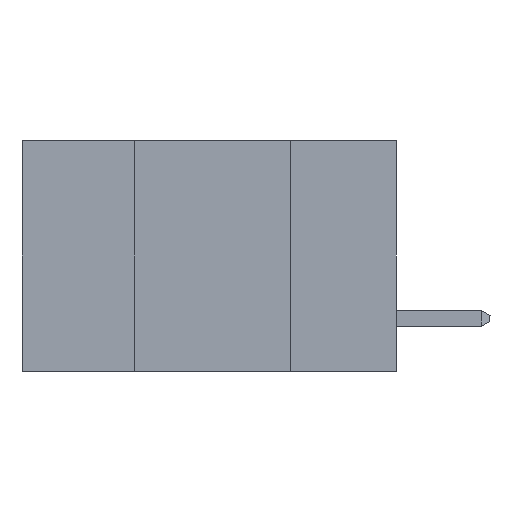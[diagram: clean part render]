
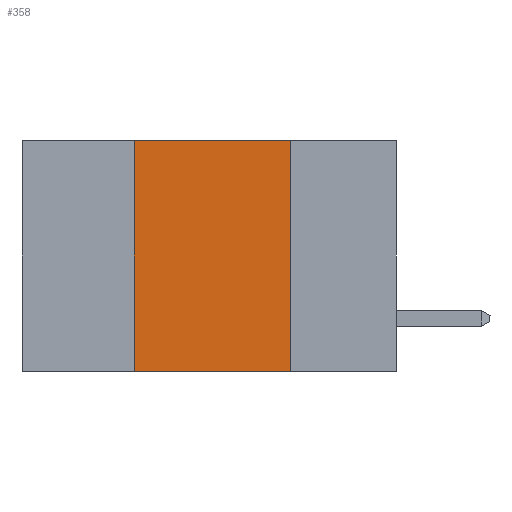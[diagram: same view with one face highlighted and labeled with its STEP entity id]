
A CAD part, left-side view. The second image highlights one B-rep face of the part: STEP entity #358.
In plain terms, the highlighted planar face has unit normal (-1, 0, 0).
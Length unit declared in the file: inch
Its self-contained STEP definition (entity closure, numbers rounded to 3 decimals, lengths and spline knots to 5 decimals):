
#358 = ADVANCED_FACE ( 'NONE', ( #4982 ), #2675, .F. ) ;
#968 = ORIENTED_EDGE ( 'NONE', *, *, #7099, .T. ) ;
#1927 = CARTESIAN_POINT ( 'NONE',  ( 0., 0.17, -0.37 ) ) ;
#2008 = CARTESIAN_POINT ( 'NONE',  ( 0., 0.6, -0.37 ) ) ;
#2015 = EDGE_CURVE ( 'NONE', #12877, #10382, #12241, .T. ) ;
#2230 = DIRECTION ( 'NONE',  ( 0., 0., 1. ) ) ;
#2251 = DIRECTION ( 'NONE',  ( 1., 0., 0. ) ) ;
#2473 = ORIENTED_EDGE ( 'NONE', *, *, #2015, .F. ) ;
#2675 = PLANE ( 'NONE',  #3673 ) ;
#2686 = CARTESIAN_POINT ( 'NONE',  ( 0., 0.17, 0. ) ) ;
#2893 = VERTEX_POINT ( 'NONE', #8122 ) ;
#3106 = DIRECTION ( 'NONE',  ( 0., -1., 0. ) ) ;
#3188 = CARTESIAN_POINT ( 'NONE',  ( 0., 0.42, -0.37 ) ) ;
#3673 = AXIS2_PLACEMENT_3D ( 'NONE', #11210, #2251, #12007 ) ;
#4173 = LINE ( 'NONE', #2008, #9363 ) ;
#4434 = LINE ( 'NONE', #12278, #9606 ) ;
#4982 = FACE_OUTER_BOUND ( 'NONE', #12709, .T. ) ;
#6560 = EDGE_CURVE ( 'NONE', #10850, #2893, #7350, .T. ) ;
#7099 = EDGE_CURVE ( 'NONE', #12877, #2893, #4173, .T. ) ;
#7350 = LINE ( 'NONE', #1927, #12438 ) ;
#7653 = ORIENTED_EDGE ( 'NONE', *, *, #9273, .F. ) ;
#8122 = CARTESIAN_POINT ( 'NONE',  ( 0., 0.17, -0.37 ) ) ;
#8143 = CARTESIAN_POINT ( 'NONE',  ( 0., 0.42, 0. ) ) ;
#8172 = DIRECTION ( 'NONE',  ( 0., 0., -1. ) ) ;
#9273 = EDGE_CURVE ( 'NONE', #10382, #10850, #4434, .T. ) ;
#9363 = VECTOR ( 'NONE', #3106, 39.37008 ) ;
#9596 = VECTOR ( 'NONE', #2230, 39.37008 ) ;
#9606 = VECTOR ( 'NONE', #11286, 39.37008 ) ;
#10382 = VERTEX_POINT ( 'NONE', #8143 ) ;
#10850 = VERTEX_POINT ( 'NONE', #2686 ) ;
#11210 = CARTESIAN_POINT ( 'NONE',  ( 0., 0.6, 0. ) ) ;
#11286 = DIRECTION ( 'NONE',  ( 0., -1., 0. ) ) ;
#12007 = DIRECTION ( 'NONE',  ( 0., 0., -1. ) ) ;
#12106 = ORIENTED_EDGE ( 'NONE', *, *, #6560, .F. ) ;
#12241 = LINE ( 'NONE', #13274, #9596 ) ;
#12278 = CARTESIAN_POINT ( 'NONE',  ( 0., 0.6, 0. ) ) ;
#12438 = VECTOR ( 'NONE', #8172, 39.37008 ) ;
#12709 = EDGE_LOOP ( 'NONE', ( #12106, #7653, #2473, #968 ) ) ;
#12877 = VERTEX_POINT ( 'NONE', #3188 ) ;
#13274 = CARTESIAN_POINT ( 'NONE',  ( 0., 0.42, -0.37 ) ) ;
